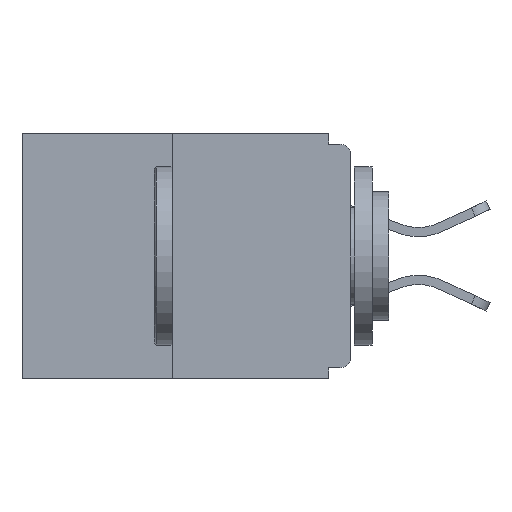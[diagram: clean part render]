
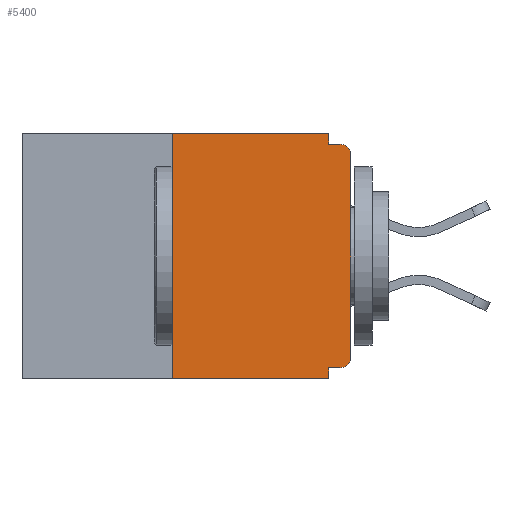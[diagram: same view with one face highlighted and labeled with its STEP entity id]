
A CAD part, left-side view. The second image highlights one B-rep face of the part: STEP entity #5400.
In plain terms, the highlighted planar face has unit normal (-1, 0, 0).
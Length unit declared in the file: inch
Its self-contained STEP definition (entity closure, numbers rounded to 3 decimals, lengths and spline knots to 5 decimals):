
#1 = VERTEX_POINT ( 'NONE', #748 ) ;
#438 = LINE ( 'NONE', #3484, #2463 ) ;
#452 = VERTEX_POINT ( 'NONE', #5317 ) ;
#745 = CARTESIAN_POINT ( 'NONE',  ( 0., 0., -0.03 ) ) ;
#748 = CARTESIAN_POINT ( 'NONE',  ( 0., 0.25, -0.343 ) ) ;
#1368 = CARTESIAN_POINT ( 'NONE',  ( 0., 0.46, 0. ) ) ;
#1369 = EDGE_CURVE ( 'NONE', #1, #6161, #8324, .T. ) ;
#1441 = LINE ( 'NONE', #12296, #9121 ) ;
#1575 = DIRECTION ( 'NONE',  ( -1., 0., 0. ) ) ;
#2031 = CARTESIAN_POINT ( 'NONE',  ( 0., 0.015, -0.313 ) ) ;
#2186 = AXIS2_PLACEMENT_3D ( 'NONE', #2031, #6717, #10172 ) ;
#2382 = DIRECTION ( 'NONE',  ( 0., 1., 0. ) ) ;
#2463 = VECTOR ( 'NONE', #10367, 39.37008 ) ;
#2479 = CARTESIAN_POINT ( 'NONE',  ( 0., 0., -0.328 ) ) ;
#2586 = VECTOR ( 'NONE', #4300, 39.37008 ) ;
#2592 = EDGE_CURVE ( 'NONE', #14673, #14028, #9764, .T. ) ;
#2719 = CARTESIAN_POINT ( 'NONE',  ( 0., 0.015, -0.03 ) ) ;
#2725 = EDGE_CURVE ( 'NONE', #1, #452, #12820, .T. ) ;
#2903 = VERTEX_POINT ( 'NONE', #8690 ) ;
#3202 = DIRECTION ( 'NONE',  ( 0., 0., -1. ) ) ;
#3484 = CARTESIAN_POINT ( 'NONE',  ( 0., 0.031, -0.343 ) ) ;
#3749 = DIRECTION ( 'NONE',  ( 0., 0., -1. ) ) ;
#3885 = LINE ( 'NONE', #10316, #10788 ) ;
#3983 = EDGE_CURVE ( 'NONE', #10359, #2903, #3885, .T. ) ;
#4090 = ORIENTED_EDGE ( 'NONE', *, *, #13449, .T. ) ;
#4149 = CARTESIAN_POINT ( 'NONE',  ( 0., 0.031, -0.343 ) ) ;
#4300 = DIRECTION ( 'NONE',  ( 0., 0., 1. ) ) ;
#4451 = ORIENTED_EDGE ( 'NONE', *, *, #13948, .F. ) ;
#4748 = VERTEX_POINT ( 'NONE', #7282 ) ;
#5008 = ORIENTED_EDGE ( 'NONE', *, *, #2725, .F. ) ;
#5050 = CIRCLE ( 'NONE', #13636, 0.015 ) ;
#5172 = ORIENTED_EDGE ( 'NONE', *, *, #3983, .F. ) ;
#5317 = CARTESIAN_POINT ( 'NONE',  ( 0., 0.25, 0. ) ) ;
#5356 = LINE ( 'NONE', #2479, #12615 ) ;
#5400 = ADVANCED_FACE ( 'NONE', ( #6382 ), #10234, .F. ) ;
#5785 = ORIENTED_EDGE ( 'NONE', *, *, #1369, .T. ) ;
#6005 = DIRECTION ( 'NONE',  ( 0., -1., 0. ) ) ;
#6161 = VERTEX_POINT ( 'NONE', #4149 ) ;
#6382 = FACE_OUTER_BOUND ( 'NONE', #15004, .T. ) ;
#6717 = DIRECTION ( 'NONE',  ( -1., 0., 0. ) ) ;
#7022 = DIRECTION ( 'NONE',  ( 0., 0., 1. ) ) ;
#7282 = CARTESIAN_POINT ( 'NONE',  ( 0., 0.031, -0.328 ) ) ;
#7696 = ORIENTED_EDGE ( 'NONE', *, *, #13724, .F. ) ;
#7848 = DIRECTION ( 'NONE',  ( 0., 0., -1. ) ) ;
#7990 = VERTEX_POINT ( 'NONE', #745 ) ;
#8035 = DIRECTION ( 'NONE',  ( 0., -1., 0. ) ) ;
#8324 = LINE ( 'NONE', #13522, #11746 ) ;
#8365 = ORIENTED_EDGE ( 'NONE', *, *, #2592, .T. ) ;
#8690 = CARTESIAN_POINT ( 'NONE',  ( 0., 0.015, -0.015 ) ) ;
#9022 = VECTOR ( 'NONE', #6005, 39.37008 ) ;
#9061 = CARTESIAN_POINT ( 'NONE',  ( 0., 0.031, 0. ) ) ;
#9063 = CARTESIAN_POINT ( 'NONE',  ( 0., 0., -0.313 ) ) ;
#9121 = VECTOR ( 'NONE', #3202, 39.37008 ) ;
#9183 = CARTESIAN_POINT ( 'NONE',  ( 0., 0.031, -0.015 ) ) ;
#9398 = VECTOR ( 'NONE', #7022, 39.37008 ) ;
#9517 = CARTESIAN_POINT ( 'NONE',  ( 0., 0.25, 0. ) ) ;
#9712 = AXIS2_PLACEMENT_3D ( 'NONE', #13612, #13663, #7848 ) ;
#9764 = CIRCLE ( 'NONE', #2186, 0.015 ) ;
#10059 = DIRECTION ( 'NONE',  ( 0., -1., 0. ) ) ;
#10172 = DIRECTION ( 'NONE',  ( 0., 0., -1. ) ) ;
#10234 = PLANE ( 'NONE',  #9712 ) ;
#10316 = CARTESIAN_POINT ( 'NONE',  ( 0., 0., -0.015 ) ) ;
#10359 = VERTEX_POINT ( 'NONE', #9183 ) ;
#10367 = DIRECTION ( 'NONE',  ( 0., 0., -1. ) ) ;
#10788 = VECTOR ( 'NONE', #8035, 39.37008 ) ;
#10994 = LINE ( 'NONE', #1368, #9022 ) ;
#11413 = ORIENTED_EDGE ( 'NONE', *, *, #13657, .T. ) ;
#11746 = VECTOR ( 'NONE', #10059, 39.37008 ) ;
#12064 = CARTESIAN_POINT ( 'NONE',  ( 0., 0.015, -0.328 ) ) ;
#12296 = CARTESIAN_POINT ( 'NONE',  ( 0., 0.031, 0. ) ) ;
#12322 = EDGE_CURVE ( 'NONE', #14221, #10359, #1441, .T. ) ;
#12420 = CARTESIAN_POINT ( 'NONE',  ( 0., 0., 0. ) ) ;
#12615 = VECTOR ( 'NONE', #2382, 39.37008 ) ;
#12820 = LINE ( 'NONE', #9517, #9398 ) ;
#13250 = ORIENTED_EDGE ( 'NONE', *, *, #12322, .F. ) ;
#13449 = EDGE_CURVE ( 'NONE', #7990, #2903, #5050, .T. ) ;
#13522 = CARTESIAN_POINT ( 'NONE',  ( 0., 0.46, -0.343 ) ) ;
#13612 = CARTESIAN_POINT ( 'NONE',  ( 0., 0.46, 0. ) ) ;
#13636 = AXIS2_PLACEMENT_3D ( 'NONE', #2719, #1575, #3749 ) ;
#13644 = LINE ( 'NONE', #12420, #2586 ) ;
#13657 = EDGE_CURVE ( 'NONE', #14028, #7990, #13644, .T. ) ;
#13663 = DIRECTION ( 'NONE',  ( 1., 0., 0. ) ) ;
#13724 = EDGE_CURVE ( 'NONE', #4748, #6161, #438, .T. ) ;
#13948 = EDGE_CURVE ( 'NONE', #452, #14221, #10994, .T. ) ;
#14028 = VERTEX_POINT ( 'NONE', #9063 ) ;
#14049 = ORIENTED_EDGE ( 'NONE', *, *, #14108, .F. ) ;
#14108 = EDGE_CURVE ( 'NONE', #14673, #4748, #5356, .T. ) ;
#14221 = VERTEX_POINT ( 'NONE', #9061 ) ;
#14673 = VERTEX_POINT ( 'NONE', #12064 ) ;
#15004 = EDGE_LOOP ( 'NONE', ( #4451, #5008, #5785, #7696, #14049, #8365, #11413, #4090, #5172, #13250 ) ) ;
